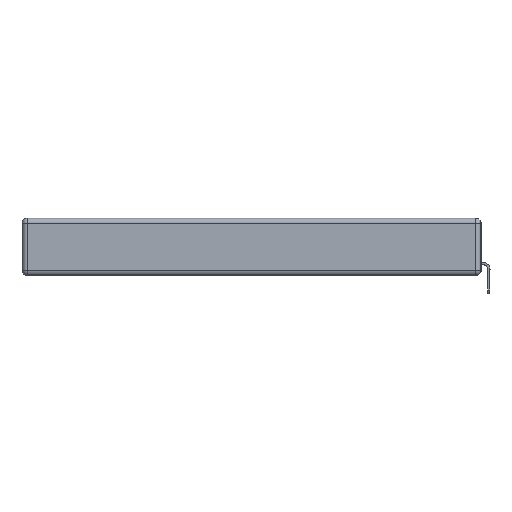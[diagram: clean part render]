
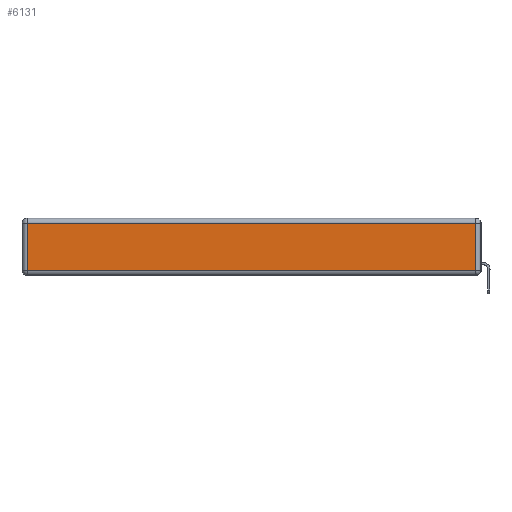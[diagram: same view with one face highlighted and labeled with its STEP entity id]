
A CAD part, left-side view. The second image highlights one B-rep face of the part: STEP entity #6131.
In plain terms, the highlighted planar face has unit normal (-1, 0, 0).
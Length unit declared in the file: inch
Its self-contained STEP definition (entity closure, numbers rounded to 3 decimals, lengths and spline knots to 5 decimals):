
#643 = VECTOR ( 'NONE', #8025, 39.37008 ) ;
#758 = CARTESIAN_POINT ( 'NONE',  ( 0., 2.72, -0.03 ) ) ;
#771 = DIRECTION ( 'NONE',  ( 0., 1., 0. ) ) ;
#846 = CARTESIAN_POINT ( 'NONE',  ( 0., 0., -0.313 ) ) ;
#1328 = CARTESIAN_POINT ( 'NONE',  ( 0., 0., -0.343 ) ) ;
#1369 = ORIENTED_EDGE ( 'NONE', *, *, #5381, .T. ) ;
#1385 = CARTESIAN_POINT ( 'NONE',  ( 0., 2.72, -0.313 ) ) ;
#1704 = CARTESIAN_POINT ( 'NONE',  ( 0., 2.75, -0.03 ) ) ;
#2201 = VERTEX_POINT ( 'NONE', #9345 ) ;
#2262 = CARTESIAN_POINT ( 'NONE',  ( 0., 2.72, -0.343 ) ) ;
#2322 = LINE ( 'NONE', #2262, #12550 ) ;
#3014 = VECTOR ( 'NONE', #771, 39.37008 ) ;
#3445 = EDGE_CURVE ( 'NONE', #10717, #13129, #2322, .T. ) ;
#3503 = VECTOR ( 'NONE', #5516, 39.37008 ) ;
#3850 = CARTESIAN_POINT ( 'NONE',  ( 0., 0.03, -0.313 ) ) ;
#4685 = ORIENTED_EDGE ( 'NONE', *, *, #3445, .T. ) ;
#5118 = EDGE_CURVE ( 'NONE', #13129, #7082, #5936, .T. ) ;
#5381 = EDGE_CURVE ( 'NONE', #2201, #10717, #8740, .T. ) ;
#5421 = DIRECTION ( 'NONE',  ( -1., 0., 0. ) ) ;
#5516 = DIRECTION ( 'NONE',  ( 0., 0., 1. ) ) ;
#5674 = EDGE_LOOP ( 'NONE', ( #12702, #13207, #1369, #4685 ) ) ;
#5936 = LINE ( 'NONE', #846, #643 ) ;
#6131 = ADVANCED_FACE ( 'NONE', ( #11752 ), #8438, .T. ) ;
#7082 = VERTEX_POINT ( 'NONE', #3850 ) ;
#7090 = AXIS2_PLACEMENT_3D ( 'NONE', #1328, #5421, #11553 ) ;
#8025 = DIRECTION ( 'NONE',  ( 0., -1., 0. ) ) ;
#8225 = EDGE_CURVE ( 'NONE', #7082, #2201, #11590, .T. ) ;
#8438 = PLANE ( 'NONE',  #7090 ) ;
#8598 = CARTESIAN_POINT ( 'NONE',  ( 0., 0.03, -0.343 ) ) ;
#8740 = LINE ( 'NONE', #1704, #3014 ) ;
#9345 = CARTESIAN_POINT ( 'NONE',  ( 0., 0.03, -0.03 ) ) ;
#10402 = DIRECTION ( 'NONE',  ( 0., 0., -1. ) ) ;
#10717 = VERTEX_POINT ( 'NONE', #758 ) ;
#11553 = DIRECTION ( 'NONE',  ( 0., 0., 1. ) ) ;
#11590 = LINE ( 'NONE', #8598, #3503 ) ;
#11752 = FACE_OUTER_BOUND ( 'NONE', #5674, .T. ) ;
#12550 = VECTOR ( 'NONE', #10402, 39.37008 ) ;
#12702 = ORIENTED_EDGE ( 'NONE', *, *, #5118, .T. ) ;
#13129 = VERTEX_POINT ( 'NONE', #1385 ) ;
#13207 = ORIENTED_EDGE ( 'NONE', *, *, #8225, .T. ) ;
